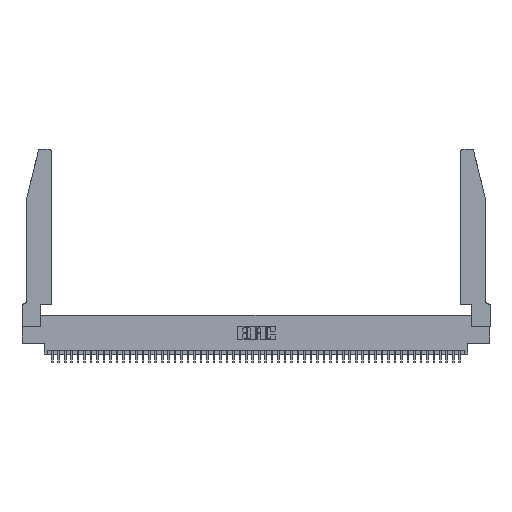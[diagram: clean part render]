
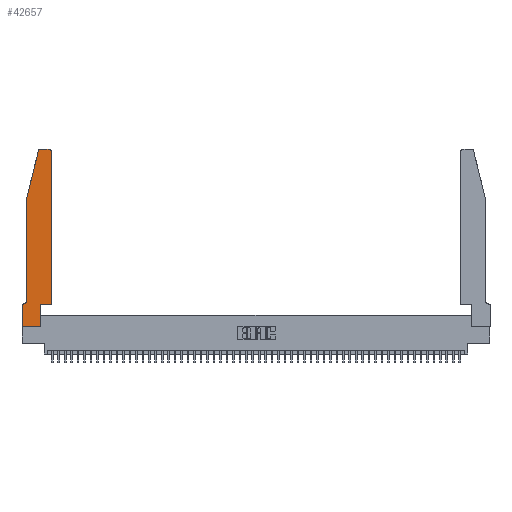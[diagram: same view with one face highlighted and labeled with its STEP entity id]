
A CAD part, top view. The second image highlights one B-rep face of the part: STEP entity #42657.
In plain terms, the highlighted planar face has unit normal (0, 0, 1).
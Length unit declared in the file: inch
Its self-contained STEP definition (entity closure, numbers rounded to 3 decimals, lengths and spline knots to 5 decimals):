
#264 = VECTOR ( 'NONE', #39468, 39.37008 ) ;
#395 = CARTESIAN_POINT ( 'NONE',  ( 0.25487, 2.72718, 0.37 ) ) ;
#2040 = VECTOR ( 'NONE', #41999, 39.37008 ) ;
#2321 = VERTEX_POINT ( 'NONE', #4814 ) ;
#2836 = ORIENTED_EDGE ( 'NONE', *, *, #44770, .T. ) ;
#3078 = ORIENTED_EDGE ( 'NONE', *, *, #12633, .T. ) ;
#3340 = CARTESIAN_POINT ( 'NONE',  ( 0.0755, 2., 0.37 ) ) ;
#4322 = EDGE_CURVE ( 'NONE', #32530, #36371, #37722, .T. ) ;
#4814 = CARTESIAN_POINT ( 'NONE',  ( 0.0755, 0.42, 0.37 ) ) ;
#5171 = CARTESIAN_POINT ( 'NONE',  ( 0.4205, 2.72, 0.37 ) ) ;
#5548 = EDGE_CURVE ( 'NONE', #45446, #30636, #25570, .T. ) ;
#7113 = CARTESIAN_POINT ( 'NONE',  ( 0.0055, 0.35, 0.37 ) ) ;
#7521 = DIRECTION ( 'NONE',  ( 0., 0., -1. ) ) ;
#7673 = LINE ( 'NONE', #17440, #34816 ) ;
#7879 = CARTESIAN_POINT ( 'NONE',  ( 0.0055, 0.42, 0.37 ) ) ;
#8147 = CIRCLE ( 'NONE', #50872, 0.03 ) ;
#9050 = CARTESIAN_POINT ( 'NONE',  ( 0.0755, 0.35, 0.37 ) ) ;
#9233 = DIRECTION ( 'NONE',  ( 1., 0., 0. ) ) ;
#10621 = ORIENTED_EDGE ( 'NONE', *, *, #47801, .T. ) ;
#10790 = LINE ( 'NONE', #37537, #2040 ) ;
#11046 = ORIENTED_EDGE ( 'NONE', *, *, #37350, .T. ) ;
#11213 = AXIS2_PLACEMENT_3D ( 'NONE', #7879, #7521, #43897 ) ;
#11496 = CARTESIAN_POINT ( 'NONE',  ( 0., 0.35, 0.37 ) ) ;
#11534 = CARTESIAN_POINT ( 'NONE',  ( 0., 0.35, 0.37 ) ) ;
#12015 = ORIENTED_EDGE ( 'NONE', *, *, #45911, .T. ) ;
#12633 = EDGE_CURVE ( 'NONE', #46436, #23998, #7673, .T. ) ;
#13132 = CARTESIAN_POINT ( 'NONE',  ( 0.284, 2.75, 0.37 ) ) ;
#13577 = AXIS2_PLACEMENT_3D ( 'NONE', #11534, #39771, #15616 ) ;
#13915 = DIRECTION ( 'NONE',  ( 0., 0., 1. ) ) ;
#14476 = DIRECTION ( 'NONE',  ( 0., -1., 0. ) ) ;
#15258 = LINE ( 'NONE', #9050, #20879 ) ;
#15616 = DIRECTION ( 'NONE',  ( 1., 0., 0. ) ) ;
#17440 = CARTESIAN_POINT ( 'NONE',  ( 0.2605, 2.75, 0.37 ) ) ;
#18295 = CARTESIAN_POINT ( 'NONE',  ( 0.284, 2.72, 0.37 ) ) ;
#19832 = EDGE_CURVE ( 'NONE', #23998, #51047, #38107, .T. ) ;
#20482 = DIRECTION ( 'NONE',  ( -1., 0., 0. ) ) ;
#20879 = VECTOR ( 'NONE', #20482, 39.37008 ) ;
#20978 = VERTEX_POINT ( 'NONE', #21714 ) ;
#21714 = CARTESIAN_POINT ( 'NONE',  ( 0.0755, 2., 0.37 ) ) ;
#21830 = DIRECTION ( 'NONE',  ( -1., 0., 0. ) ) ;
#22132 = DIRECTION ( 'NONE',  ( 0., 1., 0. ) ) ;
#22313 = CARTESIAN_POINT ( 'NONE',  ( 0.4505, 0.35, 0.37 ) ) ;
#22717 = DIRECTION ( 'NONE',  ( 0., 1., 0. ) ) ;
#23392 = CARTESIAN_POINT ( 'NONE',  ( 0.0755, 2., 0.37 ) ) ;
#23998 = VERTEX_POINT ( 'NONE', #13132 ) ;
#24445 = VECTOR ( 'NONE', #22132, 39.37008 ) ;
#25570 = LINE ( 'NONE', #26771, #46435 ) ;
#26671 = CARTESIAN_POINT ( 'NONE',  ( 0.2865, 0., 0.37 ) ) ;
#26771 = CARTESIAN_POINT ( 'NONE',  ( 0.2865, 0.35, 0.37 ) ) ;
#27048 = VERTEX_POINT ( 'NONE', #11496 ) ;
#27134 = CARTESIAN_POINT ( 'NONE',  ( 0.4505, 0.35, 0.37 ) ) ;
#27924 = PLANE ( 'NONE',  #13577 ) ;
#28871 = AXIS2_PLACEMENT_3D ( 'NONE', #18295, #13915, #30102 ) ;
#28937 = ORIENTED_EDGE ( 'NONE', *, *, #40881, .T. ) ;
#30102 = DIRECTION ( 'NONE',  ( 1., 0., 0. ) ) ;
#30154 = VERTEX_POINT ( 'NONE', #34601 ) ;
#30636 = VERTEX_POINT ( 'NONE', #33841 ) ;
#31072 = ORIENTED_EDGE ( 'NONE', *, *, #4322, .T. ) ;
#31185 = DIRECTION ( 'NONE',  ( -0.239, -0.971, 0. ) ) ;
#32530 = VERTEX_POINT ( 'NONE', #36025 ) ;
#33112 = ORIENTED_EDGE ( 'NONE', *, *, #50806, .T. ) ;
#33372 = DIRECTION ( 'NONE',  ( 0., 0., 1. ) ) ;
#33523 = VERTEX_POINT ( 'NONE', #7113 ) ;
#33622 = ORIENTED_EDGE ( 'NONE', *, *, #19832, .T. ) ;
#33841 = CARTESIAN_POINT ( 'NONE',  ( 0.2865, 0.35, 0.37 ) ) ;
#34226 = CARTESIAN_POINT ( 'NONE',  ( 0., 0., 0.37 ) ) ;
#34601 = CARTESIAN_POINT ( 'NONE',  ( 0., 0., 0.37 ) ) ;
#34607 = FACE_OUTER_BOUND ( 'NONE', #41032, .T. ) ;
#34816 = VECTOR ( 'NONE', #21830, 39.37008 ) ;
#35615 = DIRECTION ( 'NONE',  ( 1., 0., 0. ) ) ;
#36025 = CARTESIAN_POINT ( 'NONE',  ( 0.4505, 0.35, 0.37 ) ) ;
#36138 = ORIENTED_EDGE ( 'NONE', *, *, #5548, .T. ) ;
#36236 = ORIENTED_EDGE ( 'NONE', *, *, #37280, .T. ) ;
#36371 = VERTEX_POINT ( 'NONE', #41211 ) ;
#37280 = EDGE_CURVE ( 'NONE', #27048, #30154, #43178, .T. ) ;
#37350 = EDGE_CURVE ( 'NONE', #51047, #20978, #48118, .T. ) ;
#37537 = CARTESIAN_POINT ( 'NONE',  ( 0., 0., 0.37 ) ) ;
#37722 = LINE ( 'NONE', #22313, #24445 ) ;
#38107 = CIRCLE ( 'NONE', #28871, 0.03 ) ;
#38721 = VECTOR ( 'NONE', #14476, 39.37008 ) ;
#39468 = DIRECTION ( 'NONE',  ( 0., -1., 0. ) ) ;
#39771 = DIRECTION ( 'NONE',  ( 0., 0., 1. ) ) ;
#40678 = LINE ( 'NONE', #27134, #43846 ) ;
#40881 = EDGE_CURVE ( 'NONE', #30154, #45446, #10790, .T. ) ;
#41032 = EDGE_LOOP ( 'NONE', ( #3078, #33622, #11046, #48421, #2836, #12015, #36236, #28937, #36138, #33112, #31072, #10621 ) ) ;
#41211 = CARTESIAN_POINT ( 'NONE',  ( 0.4505, 2.72, 0.37 ) ) ;
#41999 = DIRECTION ( 'NONE',  ( 1., 0., 0. ) ) ;
#42657 = ADVANCED_FACE ( 'NONE', ( #34607 ), #27924, .T. ) ;
#43178 = LINE ( 'NONE', #34226, #38721 ) ;
#43784 = VECTOR ( 'NONE', #31185, 39.37008 ) ;
#43846 = VECTOR ( 'NONE', #35615, 39.37008 ) ;
#43897 = DIRECTION ( 'NONE',  ( -1., 0., 0. ) ) ;
#43928 = EDGE_CURVE ( 'NONE', #20978, #2321, #50060, .T. ) ;
#44770 = EDGE_CURVE ( 'NONE', #2321, #33523, #46846, .T. ) ;
#45446 = VERTEX_POINT ( 'NONE', #26671 ) ;
#45911 = EDGE_CURVE ( 'NONE', #33523, #27048, #15258, .T. ) ;
#46435 = VECTOR ( 'NONE', #22717, 39.37008 ) ;
#46436 = VERTEX_POINT ( 'NONE', #48128 ) ;
#46846 = CIRCLE ( 'NONE', #11213, 0.07 ) ;
#47801 = EDGE_CURVE ( 'NONE', #36371, #46436, #8147, .T. ) ;
#48118 = LINE ( 'NONE', #3340, #43784 ) ;
#48128 = CARTESIAN_POINT ( 'NONE',  ( 0.4205, 2.75, 0.37 ) ) ;
#48421 = ORIENTED_EDGE ( 'NONE', *, *, #43928, .T. ) ;
#50060 = LINE ( 'NONE', #23392, #264 ) ;
#50806 = EDGE_CURVE ( 'NONE', #30636, #32530, #40678, .T. ) ;
#50872 = AXIS2_PLACEMENT_3D ( 'NONE', #5171, #33372, #9233 ) ;
#51047 = VERTEX_POINT ( 'NONE', #395 ) ;
